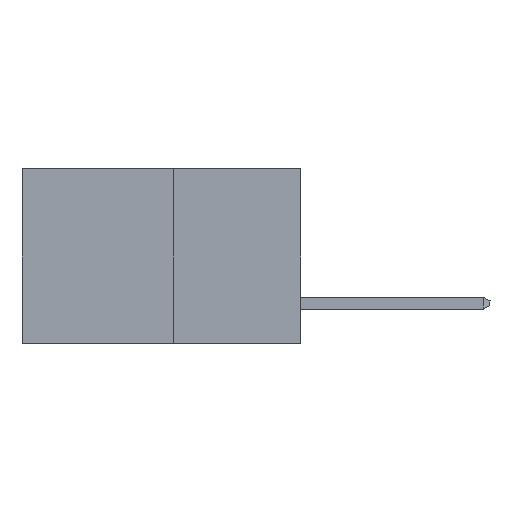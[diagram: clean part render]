
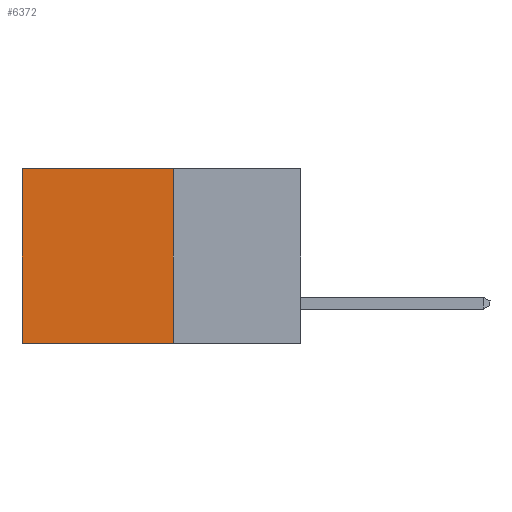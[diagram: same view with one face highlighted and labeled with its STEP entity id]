
A CAD part, left-side view. The second image highlights one B-rep face of the part: STEP entity #6372.
In plain terms, the highlighted planar face has unit normal (-1, 0, 0).
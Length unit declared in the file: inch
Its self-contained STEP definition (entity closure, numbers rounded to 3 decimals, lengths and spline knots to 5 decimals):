
#171 = EDGE_CURVE ( 'NONE', #8400, #2012, #952, .T. ) ;
#521 = ORIENTED_EDGE ( 'NONE', *, *, #1756, .T. ) ;
#661 = VECTOR ( 'NONE', #2109, 39.37008 ) ;
#896 = ORIENTED_EDGE ( 'NONE', *, *, #8641, .F. ) ;
#952 = LINE ( 'NONE', #4213, #5673 ) ;
#976 = ORIENTED_EDGE ( 'NONE', *, *, #7424, .F. ) ;
#1075 = ORIENTED_EDGE ( 'NONE', *, *, #171, .T. ) ;
#1756 = EDGE_CURVE ( 'NONE', #3073, #8400, #5209, .T. ) ;
#1916 = CARTESIAN_POINT ( 'NONE',  ( 0.277, 0.27, 0. ) ) ;
#2012 = VERTEX_POINT ( 'NONE', #9778 ) ;
#2109 = DIRECTION ( 'NONE',  ( 0., 1., 0. ) ) ;
#2311 = DIRECTION ( 'NONE',  ( 0., 1., 0. ) ) ;
#2807 = CARTESIAN_POINT ( 'NONE',  ( 0.277, 0.27, -0.37 ) ) ;
#3073 = VERTEX_POINT ( 'NONE', #10024 ) ;
#3764 = DIRECTION ( 'NONE',  ( 0., 0., -1. ) ) ;
#4104 = EDGE_LOOP ( 'NONE', ( #1075, #976, #896, #521 ) ) ;
#4213 = CARTESIAN_POINT ( 'NONE',  ( 0.277, 0.59, -0.37 ) ) ;
#4485 = FACE_OUTER_BOUND ( 'NONE', #4104, .T. ) ;
#4952 = VECTOR ( 'NONE', #2311, 39.37008 ) ;
#5209 = LINE ( 'NONE', #1916, #4952 ) ;
#5673 = VECTOR ( 'NONE', #7633, 39.37008 ) ;
#5773 = VERTEX_POINT ( 'NONE', #11397 ) ;
#5948 = LINE ( 'NONE', #8329, #661 ) ;
#6372 = ADVANCED_FACE ( 'NONE', ( #4485 ), #11236, .F. ) ;
#6829 = LINE ( 'NONE', #2807, #8836 ) ;
#7095 = DIRECTION ( 'NONE',  ( 0., 0., -1. ) ) ;
#7119 = DIRECTION ( 'NONE',  ( 1., 0., 0. ) ) ;
#7424 = EDGE_CURVE ( 'NONE', #5773, #2012, #5948, .T. ) ;
#7524 = AXIS2_PLACEMENT_3D ( 'NONE', #11240, #7119, #7095 ) ;
#7633 = DIRECTION ( 'NONE',  ( 0., 0., -1. ) ) ;
#8329 = CARTESIAN_POINT ( 'NONE',  ( 0.277, 0.27, -0.37 ) ) ;
#8400 = VERTEX_POINT ( 'NONE', #8626 ) ;
#8626 = CARTESIAN_POINT ( 'NONE',  ( 0.277, 0.59, 0. ) ) ;
#8641 = EDGE_CURVE ( 'NONE', #3073, #5773, #6829, .T. ) ;
#8836 = VECTOR ( 'NONE', #3764, 39.37008 ) ;
#9778 = CARTESIAN_POINT ( 'NONE',  ( 0.277, 0.59, -0.37 ) ) ;
#10024 = CARTESIAN_POINT ( 'NONE',  ( 0.277, 0.27, 0. ) ) ;
#11236 = PLANE ( 'NONE',  #7524 ) ;
#11240 = CARTESIAN_POINT ( 'NONE',  ( 0.277, 0.27, -0.37 ) ) ;
#11397 = CARTESIAN_POINT ( 'NONE',  ( 0.277, 0.27, -0.37 ) ) ;
